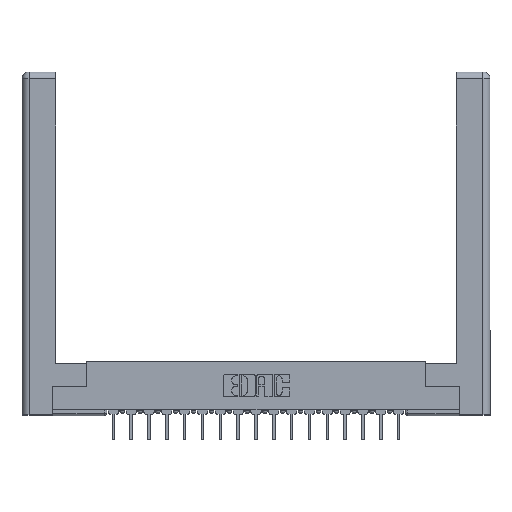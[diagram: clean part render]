
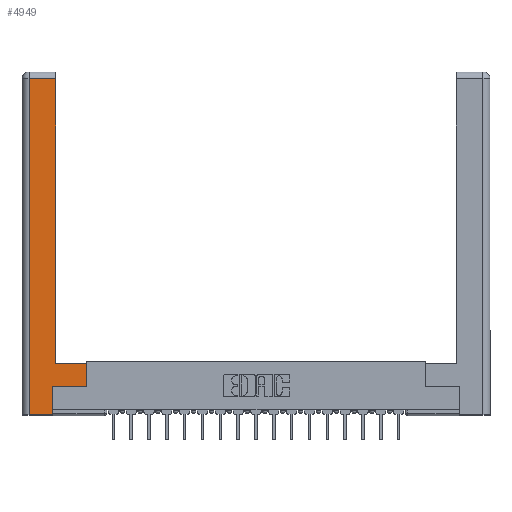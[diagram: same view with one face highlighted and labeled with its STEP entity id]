
A CAD part, top view. The second image highlights one B-rep face of the part: STEP entity #4949.
In plain terms, the highlighted planar face has unit normal (0, 0, 1).
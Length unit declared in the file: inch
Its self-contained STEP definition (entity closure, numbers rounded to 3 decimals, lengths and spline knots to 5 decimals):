
#283 = CARTESIAN_POINT ( 'NONE',  ( 0.565, 0.45, 0. ) ) ;
#462 = ORIENTED_EDGE ( 'NONE', *, *, #15806, .T. ) ;
#986 = DIRECTION ( 'NONE',  ( 1., 0., 0. ) ) ;
#1019 = VECTOR ( 'NONE', #3649, 39.37008 ) ;
#1035 = VECTOR ( 'NONE', #3395, 39.37008 ) ;
#1074 = VERTEX_POINT ( 'NONE', #18930 ) ;
#1983 = LINE ( 'NONE', #9965, #4664 ) ;
#2404 = CARTESIAN_POINT ( 'NONE',  ( 0.295, 2.94, 0. ) ) ;
#2415 = EDGE_CURVE ( 'NONE', #14394, #17851, #11282, .T. ) ;
#2450 = VERTEX_POINT ( 'NONE', #13285 ) ;
#2604 = VECTOR ( 'NONE', #11340, 39.37008 ) ;
#2681 = VERTEX_POINT ( 'NONE', #17152 ) ;
#2924 = ORIENTED_EDGE ( 'NONE', *, *, #11297, .T. ) ;
#3395 = DIRECTION ( 'NONE',  ( 0., 1., 0. ) ) ;
#3564 = DIRECTION ( 'NONE',  ( -1., 0., 0. ) ) ;
#3649 = DIRECTION ( 'NONE',  ( 0., 1., 0. ) ) ;
#4248 = VECTOR ( 'NONE', #18103, 39.37008 ) ;
#4664 = VECTOR ( 'NONE', #3564, 39.37008 ) ;
#4676 = LINE ( 'NONE', #8123, #1019 ) ;
#4949 = ADVANCED_FACE ( 'NONE', ( #18138 ), #19849, .F. ) ;
#5695 = LINE ( 'NONE', #16455, #4248 ) ;
#5825 = DIRECTION ( 'NONE',  ( 0., 0., -1. ) ) ;
#6031 = CARTESIAN_POINT ( 'NONE',  ( 0.295, 0.45, 0. ) ) ;
#6081 = LINE ( 'NONE', #11769, #7524 ) ;
#6177 = VECTOR ( 'NONE', #986, 39.37008 ) ;
#6293 = VECTOR ( 'NONE', #16562, 39.37008 ) ;
#6640 = ORIENTED_EDGE ( 'NONE', *, *, #10728, .T. ) ;
#7335 = ORIENTED_EDGE ( 'NONE', *, *, #15329, .T. ) ;
#7524 = VECTOR ( 'NONE', #14888, 39.37008 ) ;
#8100 = ORIENTED_EDGE ( 'NONE', *, *, #16949, .T. ) ;
#8123 = CARTESIAN_POINT ( 'NONE',  ( 0.295, 3., 0. ) ) ;
#8210 = EDGE_CURVE ( 'NONE', #2450, #19910, #10419, .T. ) ;
#8835 = AXIS2_PLACEMENT_3D ( 'NONE', #16686, #5825, #10495 ) ;
#9715 = VERTEX_POINT ( 'NONE', #2404 ) ;
#9965 = CARTESIAN_POINT ( 'NONE',  ( 0.0615, 2.94, 0. ) ) ;
#10419 = LINE ( 'NONE', #12841, #2604 ) ;
#10495 = DIRECTION ( 'NONE',  ( -1., 0., 0. ) ) ;
#10728 = EDGE_CURVE ( 'NONE', #19264, #9715, #4676, .T. ) ;
#11282 = LINE ( 'NONE', #18964, #1035 ) ;
#11297 = EDGE_CURVE ( 'NONE', #9715, #2450, #1983, .T. ) ;
#11340 = DIRECTION ( 'NONE',  ( 0., -1., 0. ) ) ;
#11490 = EDGE_CURVE ( 'NONE', #1074, #14394, #6081, .T. ) ;
#11565 = ORIENTED_EDGE ( 'NONE', *, *, #11490, .T. ) ;
#11769 = CARTESIAN_POINT ( 'NONE',  ( 0.565, 0.245, 0. ) ) ;
#12013 = CARTESIAN_POINT ( 'NONE',  ( 0.295, 0.45, 0. ) ) ;
#12692 = CARTESIAN_POINT ( 'NONE',  ( 0.565, 0.245, 0. ) ) ;
#12841 = CARTESIAN_POINT ( 'NONE',  ( 0.0615, 0., 0. ) ) ;
#13285 = CARTESIAN_POINT ( 'NONE',  ( 0.0615, 2.94, 0. ) ) ;
#14394 = VERTEX_POINT ( 'NONE', #12692 ) ;
#14460 = ORIENTED_EDGE ( 'NONE', *, *, #2415, .T. ) ;
#14888 = DIRECTION ( 'NONE',  ( 1., 0., 0. ) ) ;
#15169 = CARTESIAN_POINT ( 'NONE',  ( 0.265, 0., 0. ) ) ;
#15329 = EDGE_CURVE ( 'NONE', #2681, #1074, #5695, .T. ) ;
#15806 = EDGE_CURVE ( 'NONE', #19910, #2681, #17688, .T. ) ;
#16455 = CARTESIAN_POINT ( 'NONE',  ( 0.265, 0.245, 0. ) ) ;
#16562 = DIRECTION ( 'NONE',  ( -1., 0., 0. ) ) ;
#16686 = CARTESIAN_POINT ( 'NONE',  ( 0., 0., 0. ) ) ;
#16949 = EDGE_CURVE ( 'NONE', #17851, #19264, #18047, .T. ) ;
#17152 = CARTESIAN_POINT ( 'NONE',  ( 0.265, 0., 0. ) ) ;
#17688 = LINE ( 'NONE', #15169, #6177 ) ;
#17851 = VERTEX_POINT ( 'NONE', #283 ) ;
#18047 = LINE ( 'NONE', #12013, #6293 ) ;
#18103 = DIRECTION ( 'NONE',  ( 0., 1., 0. ) ) ;
#18138 = FACE_OUTER_BOUND ( 'NONE', #19506, .T. ) ;
#18216 = ORIENTED_EDGE ( 'NONE', *, *, #8210, .T. ) ;
#18930 = CARTESIAN_POINT ( 'NONE',  ( 0.265, 0.245, 0. ) ) ;
#18964 = CARTESIAN_POINT ( 'NONE',  ( 0.565, 0.45, 0. ) ) ;
#19264 = VERTEX_POINT ( 'NONE', #6031 ) ;
#19506 = EDGE_LOOP ( 'NONE', ( #6640, #2924, #18216, #462, #7335, #11565, #14460, #8100 ) ) ;
#19637 = CARTESIAN_POINT ( 'NONE',  ( 0.0615, 0., 0. ) ) ;
#19849 = PLANE ( 'NONE',  #8835 ) ;
#19910 = VERTEX_POINT ( 'NONE', #19637 ) ;
